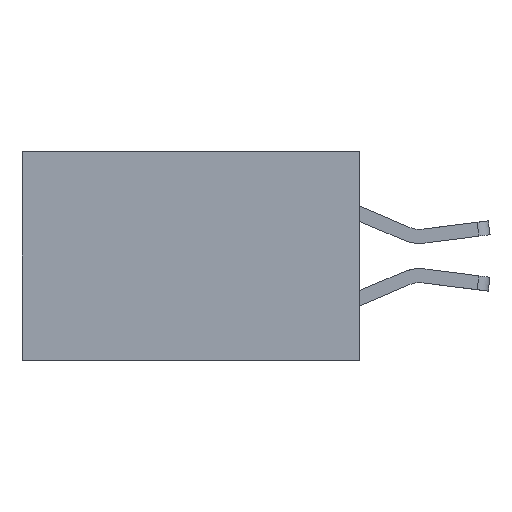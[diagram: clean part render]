
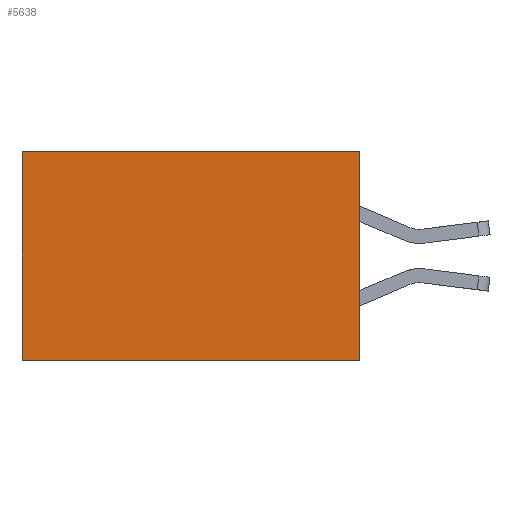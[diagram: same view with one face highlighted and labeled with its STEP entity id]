
A CAD part, left-side view. The second image highlights one B-rep face of the part: STEP entity #5638.
In plain terms, the highlighted planar face has unit normal (-1, 0, 0).
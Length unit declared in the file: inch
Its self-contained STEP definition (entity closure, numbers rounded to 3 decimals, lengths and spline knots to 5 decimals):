
#139 = ORIENTED_EDGE ( 'NONE', *, *, #9330, .F. ) ;
#685 = CARTESIAN_POINT ( 'NONE',  ( 0.2875, 0., -0.37 ) ) ;
#902 = AXIS2_PLACEMENT_3D ( 'NONE', #5140, #1210, #10062 ) ;
#915 = VERTEX_POINT ( 'NONE', #7537 ) ;
#1210 = DIRECTION ( 'NONE',  ( 1., 0., 0. ) ) ;
#1863 = LINE ( 'NONE', #685, #11426 ) ;
#2026 = DIRECTION ( 'NONE',  ( 0., 1., 0. ) ) ;
#2508 = CARTESIAN_POINT ( 'NONE',  ( 0.2875, 0., -0.37 ) ) ;
#3142 = DIRECTION ( 'NONE',  ( 0., 1., 0. ) ) ;
#3660 = ORIENTED_EDGE ( 'NONE', *, *, #5219, .F. ) ;
#3939 = EDGE_CURVE ( 'NONE', #915, #11881, #8440, .T. ) ;
#4442 = DIRECTION ( 'NONE',  ( 0., 0., -1. ) ) ;
#5140 = CARTESIAN_POINT ( 'NONE',  ( 0.2875, 0., 0. ) ) ;
#5219 = EDGE_CURVE ( 'NONE', #915, #7000, #14763, .T. ) ;
#5638 = ADVANCED_FACE ( 'NONE', ( #12681 ), #8842, .F. ) ;
#5669 = CARTESIAN_POINT ( 'NONE',  ( 0.2875, 0., 0. ) ) ;
#6278 = CARTESIAN_POINT ( 'NONE',  ( 0.2875, 0.6, -0.37 ) ) ;
#6456 = ORIENTED_EDGE ( 'NONE', *, *, #6984, .T. ) ;
#6984 = EDGE_CURVE ( 'NONE', #11881, #15185, #10950, .T. ) ;
#7000 = VERTEX_POINT ( 'NONE', #2508 ) ;
#7537 = CARTESIAN_POINT ( 'NONE',  ( 0.2875, 0., 0. ) ) ;
#7600 = EDGE_LOOP ( 'NONE', ( #6456, #139, #3660, #12622 ) ) ;
#7615 = CARTESIAN_POINT ( 'NONE',  ( 0.2875, 0.6, 0. ) ) ;
#8401 = VECTOR ( 'NONE', #4442, 39.37008 ) ;
#8440 = LINE ( 'NONE', #14904, #11610 ) ;
#8842 = PLANE ( 'NONE',  #902 ) ;
#9330 = EDGE_CURVE ( 'NONE', #7000, #15185, #1863, .T. ) ;
#10062 = DIRECTION ( 'NONE',  ( 0., 0., -1. ) ) ;
#10950 = LINE ( 'NONE', #7615, #14130 ) ;
#11426 = VECTOR ( 'NONE', #2026, 39.37008 ) ;
#11610 = VECTOR ( 'NONE', #3142, 39.37008 ) ;
#11881 = VERTEX_POINT ( 'NONE', #13869 ) ;
#12622 = ORIENTED_EDGE ( 'NONE', *, *, #3939, .T. ) ;
#12681 = FACE_OUTER_BOUND ( 'NONE', #7600, .T. ) ;
#13530 = DIRECTION ( 'NONE',  ( 0., 0., -1. ) ) ;
#13869 = CARTESIAN_POINT ( 'NONE',  ( 0.2875, 0.6, 0. ) ) ;
#14130 = VECTOR ( 'NONE', #13530, 39.37008 ) ;
#14763 = LINE ( 'NONE', #5669, #8401 ) ;
#14904 = CARTESIAN_POINT ( 'NONE',  ( 0.2875, 0., 0. ) ) ;
#15185 = VERTEX_POINT ( 'NONE', #6278 ) ;
